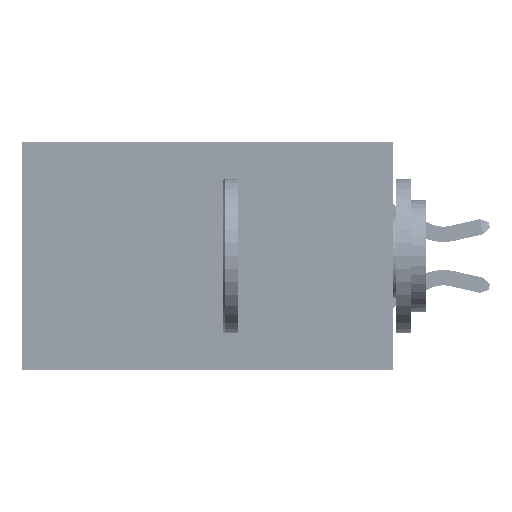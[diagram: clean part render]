
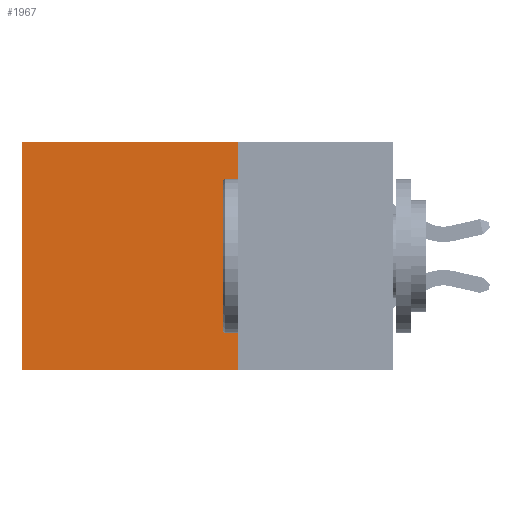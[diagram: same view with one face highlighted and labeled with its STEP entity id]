
A CAD part, left-side view. The second image highlights one B-rep face of the part: STEP entity #1967.
In plain terms, the highlighted planar face has unit normal (-1, 0, 0).
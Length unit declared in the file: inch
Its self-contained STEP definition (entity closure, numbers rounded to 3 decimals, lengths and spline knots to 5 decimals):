
#557 = VERTEX_POINT ( 'NONE', #46675 ) ;
#1133 = LINE ( 'NONE', #13290, #45720 ) ;
#1967 = ADVANCED_FACE ( 'NONE', ( #8948 ), #29876, .F. ) ;
#3381 = EDGE_CURVE ( 'NONE', #16012, #5488, #29543, .T. ) ;
#5488 = VERTEX_POINT ( 'NONE', #34593 ) ;
#5805 = CARTESIAN_POINT ( 'NONE',  ( 0.2875, 0.25, 0. ) ) ;
#8465 = VECTOR ( 'NONE', #46930, 39.37008 ) ;
#8948 = FACE_OUTER_BOUND ( 'NONE', #22405, .T. ) ;
#9077 = ORIENTED_EDGE ( 'NONE', *, *, #50099, .F. ) ;
#10065 = VECTOR ( 'NONE', #33102, 39.37008 ) ;
#10784 = ORIENTED_EDGE ( 'NONE', *, *, #26944, .T. ) ;
#13290 = CARTESIAN_POINT ( 'NONE',  ( 0.2875, 0.25, 0. ) ) ;
#14805 = CARTESIAN_POINT ( 'NONE',  ( 0.2875, 0.25, 0. ) ) ;
#16012 = VERTEX_POINT ( 'NONE', #20715 ) ;
#16373 = EDGE_CURVE ( 'NONE', #24205, #557, #23004, .T. ) ;
#18989 = ORIENTED_EDGE ( 'NONE', *, *, #3381, .F. ) ;
#20715 = CARTESIAN_POINT ( 'NONE',  ( 0.2875, 0.25, -0.37 ) ) ;
#22405 = EDGE_LOOP ( 'NONE', ( #10784, #18989, #9077, #31594 ) ) ;
#23004 = LINE ( 'NONE', #34293, #8465 ) ;
#24205 = VERTEX_POINT ( 'NONE', #14805 ) ;
#26552 = DIRECTION ( 'NONE',  ( 1., 0., 0. ) ) ;
#26944 = EDGE_CURVE ( 'NONE', #557, #5488, #38728, .T. ) ;
#29543 = LINE ( 'NONE', #36764, #10065 ) ;
#29876 = PLANE ( 'NONE',  #35968 ) ;
#31594 = ORIENTED_EDGE ( 'NONE', *, *, #16373, .T. ) ;
#33102 = DIRECTION ( 'NONE',  ( 0., 1., 0. ) ) ;
#34293 = CARTESIAN_POINT ( 'NONE',  ( 0.2875, 0.25, 0. ) ) ;
#34593 = CARTESIAN_POINT ( 'NONE',  ( 0.2875, 0.6, -0.37 ) ) ;
#34958 = VECTOR ( 'NONE', #36030, 39.37008 ) ;
#35968 = AXIS2_PLACEMENT_3D ( 'NONE', #5805, #26552, #37921 ) ;
#36030 = DIRECTION ( 'NONE',  ( 0., 0., -1. ) ) ;
#36764 = CARTESIAN_POINT ( 'NONE',  ( 0.2875, 0.25, -0.37 ) ) ;
#37921 = DIRECTION ( 'NONE',  ( 0., 0., -1. ) ) ;
#38728 = LINE ( 'NONE', #48682, #34958 ) ;
#45720 = VECTOR ( 'NONE', #49316, 39.37008 ) ;
#46675 = CARTESIAN_POINT ( 'NONE',  ( 0.2875, 0.6, 0. ) ) ;
#46930 = DIRECTION ( 'NONE',  ( 0., 1., 0. ) ) ;
#48682 = CARTESIAN_POINT ( 'NONE',  ( 0.2875, 0.6, 0. ) ) ;
#49316 = DIRECTION ( 'NONE',  ( 0., 0., -1. ) ) ;
#50099 = EDGE_CURVE ( 'NONE', #24205, #16012, #1133, .T. ) ;
